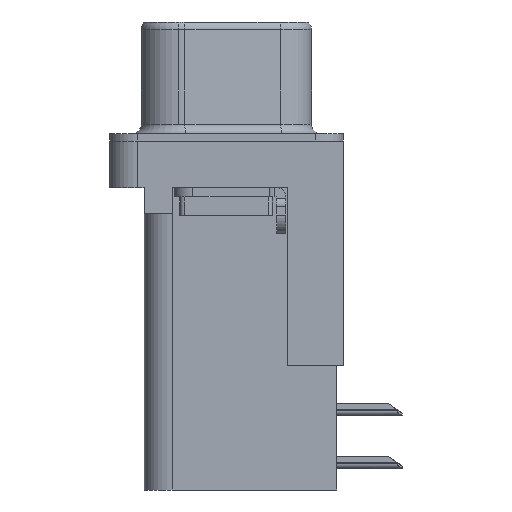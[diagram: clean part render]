
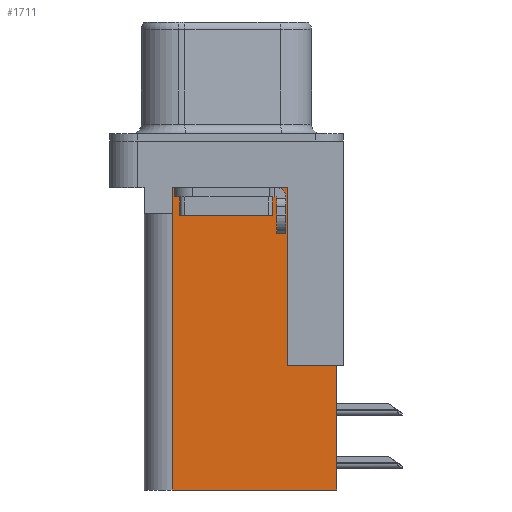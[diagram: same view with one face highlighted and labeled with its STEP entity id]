
A CAD part, left-side view. The second image highlights one B-rep face of the part: STEP entity #1711.
In plain terms, the highlighted planar face has unit normal (-1, 0, 0).
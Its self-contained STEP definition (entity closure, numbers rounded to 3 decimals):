
#9 = LINE ( 'NONE', #6671, #4184 ) ;
#197 = CARTESIAN_POINT ( 'NONE',  ( 3.7, -3.295, -2.5 ) ) ;
#324 = ORIENTED_EDGE ( 'NONE', *, *, #5021, .T. ) ;
#603 = VERTEX_POINT ( 'NONE', #18376 ) ;
#1066 = VECTOR ( 'NONE', #16138, 1000. ) ;
#1068 = EDGE_CURVE ( 'NONE', #6755, #1479, #12565, .T. ) ;
#1479 = VERTEX_POINT ( 'NONE', #3735 ) ;
#1711 = ADVANCED_FACE ( 'NONE', ( #5706 ), #18681, .F. ) ;
#1715 = DIRECTION ( 'NONE',  ( 0., 0., 1. ) ) ;
#1998 = DIRECTION ( 'NONE',  ( 0., 1., 0. ) ) ;
#2013 = DIRECTION ( 'NONE',  ( 0., 1., 0. ) ) ;
#3322 = EDGE_LOOP ( 'NONE', ( #7347, #7329, #4949, #13990, #21340, #19251, #324, #12152 ) ) ;
#3735 = CARTESIAN_POINT ( 'NONE',  ( 3.7, -5.925, -18.76 ) ) ;
#3783 = DIRECTION ( 'NONE',  ( 0., 0., -1. ) ) ;
#4184 = VECTOR ( 'NONE', #7934, 1000. ) ;
#4523 = EDGE_CURVE ( 'NONE', #14158, #17177, #18677, .T. ) ;
#4860 = EDGE_CURVE ( 'NONE', #13044, #18697, #20854, .T. ) ;
#4949 = ORIENTED_EDGE ( 'NONE', *, *, #6835, .T. ) ;
#5021 = EDGE_CURVE ( 'NONE', #6755, #13671, #9, .T. ) ;
#5706 = FACE_OUTER_BOUND ( 'NONE', #3322, .T. ) ;
#5721 = CARTESIAN_POINT ( 'NONE',  ( 3.7, -3.295, -18.76 ) ) ;
#5862 = CARTESIAN_POINT ( 'NONE',  ( 3.7, -5.925, -2. ) ) ;
#5883 = VECTOR ( 'NONE', #19197, 1000. ) ;
#6048 = DIRECTION ( 'NONE',  ( 0., 0., -1. ) ) ;
#6671 = CARTESIAN_POINT ( 'NONE',  ( 3.7, -6.295, -12.05 ) ) ;
#6755 = VERTEX_POINT ( 'NONE', #19437 ) ;
#6835 = EDGE_CURVE ( 'NONE', #18697, #17177, #20233, .T. ) ;
#6997 = CARTESIAN_POINT ( 'NONE',  ( 3.7, 0., -3.9 ) ) ;
#7329 = ORIENTED_EDGE ( 'NONE', *, *, #4860, .T. ) ;
#7347 = ORIENTED_EDGE ( 'NONE', *, *, #8832, .T. ) ;
#7934 = DIRECTION ( 'NONE',  ( 0., 1., 0. ) ) ;
#8832 = EDGE_CURVE ( 'NONE', #603, #13044, #11220, .T. ) ;
#9158 = CARTESIAN_POINT ( 'NONE',  ( 3.7, 2.925, -18.76 ) ) ;
#10444 = LINE ( 'NONE', #5721, #1066 ) ;
#10598 = CARTESIAN_POINT ( 'NONE',  ( 3.7, 2.925, -18.76 ) ) ;
#10670 = VECTOR ( 'NONE', #2013, 1000. ) ;
#11220 = LINE ( 'NONE', #197, #10670 ) ;
#12152 = ORIENTED_EDGE ( 'NONE', *, *, #14821, .T. ) ;
#12294 = CARTESIAN_POINT ( 'NONE',  ( 3.7, 2.925, -3.9 ) ) ;
#12467 = VECTOR ( 'NONE', #1715, 1000. ) ;
#12565 = LINE ( 'NONE', #5862, #21253 ) ;
#12630 = AXIS2_PLACEMENT_3D ( 'NONE', #19199, #17363, #1998 ) ;
#13009 = LINE ( 'NONE', #19150, #12467 ) ;
#13044 = VERTEX_POINT ( 'NONE', #19226 ) ;
#13671 = VERTEX_POINT ( 'NONE', #15628 ) ;
#13990 = ORIENTED_EDGE ( 'NONE', *, *, #4523, .F. ) ;
#14158 = VERTEX_POINT ( 'NONE', #10598 ) ;
#14821 = EDGE_CURVE ( 'NONE', #13671, #603, #13009, .T. ) ;
#15628 = CARTESIAN_POINT ( 'NONE',  ( 3.7, -3.295, -12.05 ) ) ;
#16138 = DIRECTION ( 'NONE',  ( 0., 1., 0. ) ) ;
#16205 = VECTOR ( 'NONE', #6048, 1000. ) ;
#17177 = VERTEX_POINT ( 'NONE', #12294 ) ;
#17363 = DIRECTION ( 'NONE',  ( 1., 0., 0. ) ) ;
#18376 = CARTESIAN_POINT ( 'NONE',  ( 3.7, -3.295, -2.5 ) ) ;
#18677 = LINE ( 'NONE', #9158, #5883 ) ;
#18681 = PLANE ( 'NONE',  #12630 ) ;
#18697 = VERTEX_POINT ( 'NONE', #19364 ) ;
#18785 = EDGE_CURVE ( 'NONE', #1479, #14158, #10444, .T. ) ;
#19150 = CARTESIAN_POINT ( 'NONE',  ( 3.7, -3.295, -18.76 ) ) ;
#19197 = DIRECTION ( 'NONE',  ( 0., 0., 1. ) ) ;
#19199 = CARTESIAN_POINT ( 'NONE',  ( 3.7, -3.295, -18.76 ) ) ;
#19226 = CARTESIAN_POINT ( 'NONE',  ( 3.7, 2.895, -2.5 ) ) ;
#19251 = ORIENTED_EDGE ( 'NONE', *, *, #1068, .F. ) ;
#19364 = CARTESIAN_POINT ( 'NONE',  ( 3.7, 2.895, -3.9 ) ) ;
#19437 = CARTESIAN_POINT ( 'NONE',  ( 3.7, -5.925, -12.05 ) ) ;
#19697 = VECTOR ( 'NONE', #22424, 1000. ) ;
#20233 = LINE ( 'NONE', #6997, #19697 ) ;
#20854 = LINE ( 'NONE', #22456, #16205 ) ;
#21253 = VECTOR ( 'NONE', #3783, 1000. ) ;
#21340 = ORIENTED_EDGE ( 'NONE', *, *, #18785, .F. ) ;
#22424 = DIRECTION ( 'NONE',  ( 0., 1., 0. ) ) ;
#22456 = CARTESIAN_POINT ( 'NONE',  ( 3.7, 2.895, -3.9 ) ) ;
